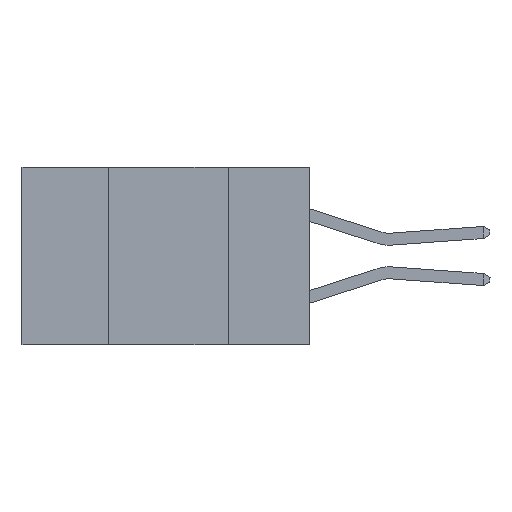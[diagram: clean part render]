
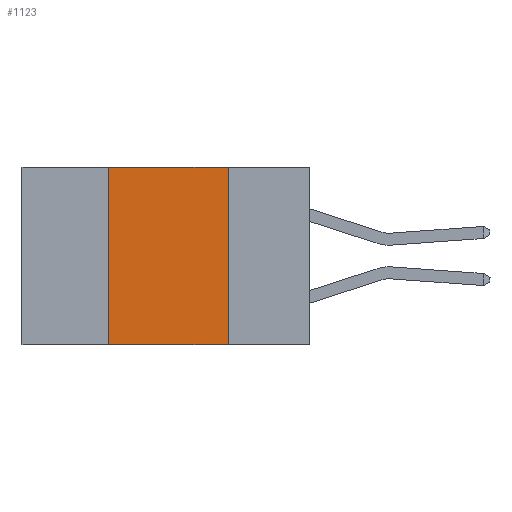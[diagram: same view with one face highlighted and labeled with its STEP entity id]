
A CAD part, left-side view. The second image highlights one B-rep face of the part: STEP entity #1123.
In plain terms, the highlighted planar face has unit normal (-1, 0, 0).
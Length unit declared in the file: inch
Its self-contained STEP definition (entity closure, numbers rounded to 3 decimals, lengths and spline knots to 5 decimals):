
#440 = EDGE_CURVE ( 'NONE', #4818, #1774, #14112, .T. ) ;
#1088 = VERTEX_POINT ( 'NONE', #5856 ) ;
#1123 = ADVANCED_FACE ( 'NONE', ( #9710 ), #17155, .F. ) ;
#1613 = DIRECTION ( 'NONE',  ( 1., 0., 0. ) ) ;
#1774 = VERTEX_POINT ( 'NONE', #9082 ) ;
#2190 = EDGE_CURVE ( 'NONE', #1774, #1088, #8299, .T. ) ;
#3814 = DIRECTION ( 'NONE',  ( 0., -1., 0. ) ) ;
#3832 = VECTOR ( 'NONE', #13308, 39.37008 ) ;
#4418 = DIRECTION ( 'NONE',  ( 0., 0., 1. ) ) ;
#4447 = CARTESIAN_POINT ( 'NONE',  ( 0., 0.42, -0.37 ) ) ;
#4528 = ORIENTED_EDGE ( 'NONE', *, *, #8418, .T. ) ;
#4580 = CARTESIAN_POINT ( 'NONE',  ( 0., 0.42, -0.37 ) ) ;
#4818 = VERTEX_POINT ( 'NONE', #18441 ) ;
#5856 = CARTESIAN_POINT ( 'NONE',  ( 0., 0.17, -0.37 ) ) ;
#6448 = EDGE_CURVE ( 'NONE', #12688, #4818, #14967, .T. ) ;
#6824 = CARTESIAN_POINT ( 'NONE',  ( 0., 0.6, -0.37 ) ) ;
#7206 = AXIS2_PLACEMENT_3D ( 'NONE', #8425, #1613, #7348 ) ;
#7348 = DIRECTION ( 'NONE',  ( 0., 0., -1. ) ) ;
#7605 = ORIENTED_EDGE ( 'NONE', *, *, #2190, .F. ) ;
#8299 = LINE ( 'NONE', #15220, #3832 ) ;
#8418 = EDGE_CURVE ( 'NONE', #12688, #1088, #16578, .T. ) ;
#8425 = CARTESIAN_POINT ( 'NONE',  ( 0., 0.6, 0. ) ) ;
#8672 = ORIENTED_EDGE ( 'NONE', *, *, #440, .F. ) ;
#8914 = VECTOR ( 'NONE', #3814, 39.37008 ) ;
#9082 = CARTESIAN_POINT ( 'NONE',  ( 0., 0.17, 0. ) ) ;
#9710 = FACE_OUTER_BOUND ( 'NONE', #15173, .T. ) ;
#9794 = VECTOR ( 'NONE', #14258, 39.37008 ) ;
#11155 = VECTOR ( 'NONE', #4418, 39.37008 ) ;
#12688 = VERTEX_POINT ( 'NONE', #4580 ) ;
#13308 = DIRECTION ( 'NONE',  ( 0., 0., -1. ) ) ;
#13695 = ORIENTED_EDGE ( 'NONE', *, *, #6448, .F. ) ;
#14112 = LINE ( 'NONE', #14155, #9794 ) ;
#14155 = CARTESIAN_POINT ( 'NONE',  ( 0., 0.6, 0. ) ) ;
#14258 = DIRECTION ( 'NONE',  ( 0., -1., 0. ) ) ;
#14967 = LINE ( 'NONE', #4447, #11155 ) ;
#15173 = EDGE_LOOP ( 'NONE', ( #7605, #8672, #13695, #4528 ) ) ;
#15220 = CARTESIAN_POINT ( 'NONE',  ( 0., 0.17, -0.37 ) ) ;
#16578 = LINE ( 'NONE', #6824, #8914 ) ;
#17155 = PLANE ( 'NONE',  #7206 ) ;
#18441 = CARTESIAN_POINT ( 'NONE',  ( 0., 0.42, 0. ) ) ;
